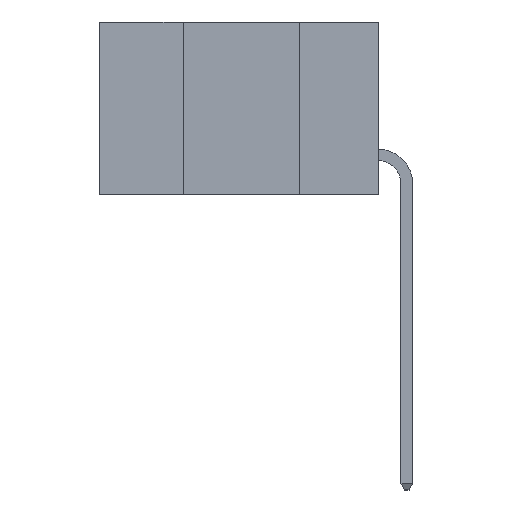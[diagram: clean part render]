
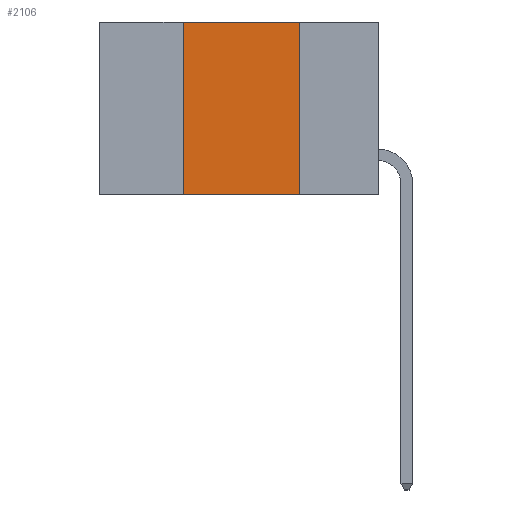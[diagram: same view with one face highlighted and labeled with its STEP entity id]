
A CAD part, left-side view. The second image highlights one B-rep face of the part: STEP entity #2106.
In plain terms, the highlighted planar face has unit normal (-1, 0, 0).
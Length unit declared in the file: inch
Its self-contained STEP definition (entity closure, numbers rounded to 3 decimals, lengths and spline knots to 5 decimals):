
#809 = CARTESIAN_POINT ( 'NONE',  ( 0., 0.17, 0. ) ) ;
#2106 = ADVANCED_FACE ( 'NONE', ( #22509 ), #7940, .F. ) ;
#2193 = VECTOR ( 'NONE', #10362, 39.37008 ) ;
#2289 = EDGE_CURVE ( 'NONE', #2570, #17910, #18387, .T. ) ;
#2570 = VERTEX_POINT ( 'NONE', #15782 ) ;
#2836 = VECTOR ( 'NONE', #19704, 39.37008 ) ;
#4310 = CARTESIAN_POINT ( 'NONE',  ( 0., 0.6, -0.37 ) ) ;
#6260 = ORIENTED_EDGE ( 'NONE', *, *, #2289, .F. ) ;
#6541 = ORIENTED_EDGE ( 'NONE', *, *, #20196, .T. ) ;
#6980 = EDGE_CURVE ( 'NONE', #23742, #12257, #15712, .T. ) ;
#7267 = DIRECTION ( 'NONE',  ( 0., 0., -1. ) ) ;
#7602 = DIRECTION ( 'NONE',  ( 1., 0., 0. ) ) ;
#7893 = ORIENTED_EDGE ( 'NONE', *, *, #13245, .F. ) ;
#7940 = PLANE ( 'NONE',  #14912 ) ;
#8281 = CARTESIAN_POINT ( 'NONE',  ( 0., 0.6, 0. ) ) ;
#9154 = DIRECTION ( 'NONE',  ( 0., 0., -1. ) ) ;
#9243 = CARTESIAN_POINT ( 'NONE',  ( 0., 0.17, -0.37 ) ) ;
#9682 = CARTESIAN_POINT ( 'NONE',  ( 0., 0.17, -0.37 ) ) ;
#10362 = DIRECTION ( 'NONE',  ( 0., -1., 0. ) ) ;
#10642 = VECTOR ( 'NONE', #9154, 39.37008 ) ;
#11562 = ORIENTED_EDGE ( 'NONE', *, *, #6980, .F. ) ;
#12257 = VERTEX_POINT ( 'NONE', #9682 ) ;
#12569 = EDGE_LOOP ( 'NONE', ( #11562, #7893, #6260, #6541 ) ) ;
#12620 = LINE ( 'NONE', #14156, #2193 ) ;
#13245 = EDGE_CURVE ( 'NONE', #17910, #23742, #12620, .T. ) ;
#14156 = CARTESIAN_POINT ( 'NONE',  ( 0., 0.6, 0. ) ) ;
#14912 = AXIS2_PLACEMENT_3D ( 'NONE', #8281, #7602, #7267 ) ;
#15410 = VECTOR ( 'NONE', #23570, 39.37008 ) ;
#15712 = LINE ( 'NONE', #9243, #10642 ) ;
#15782 = CARTESIAN_POINT ( 'NONE',  ( 0., 0.42, -0.37 ) ) ;
#17910 = VERTEX_POINT ( 'NONE', #22336 ) ;
#18387 = LINE ( 'NONE', #19572, #2836 ) ;
#19572 = CARTESIAN_POINT ( 'NONE',  ( 0., 0.42, -0.37 ) ) ;
#19704 = DIRECTION ( 'NONE',  ( 0., 0., 1. ) ) ;
#20196 = EDGE_CURVE ( 'NONE', #2570, #12257, #20508, .T. ) ;
#20508 = LINE ( 'NONE', #4310, #15410 ) ;
#22336 = CARTESIAN_POINT ( 'NONE',  ( 0., 0.42, 0. ) ) ;
#22509 = FACE_OUTER_BOUND ( 'NONE', #12569, .T. ) ;
#23570 = DIRECTION ( 'NONE',  ( 0., -1., 0. ) ) ;
#23742 = VERTEX_POINT ( 'NONE', #809 ) ;
